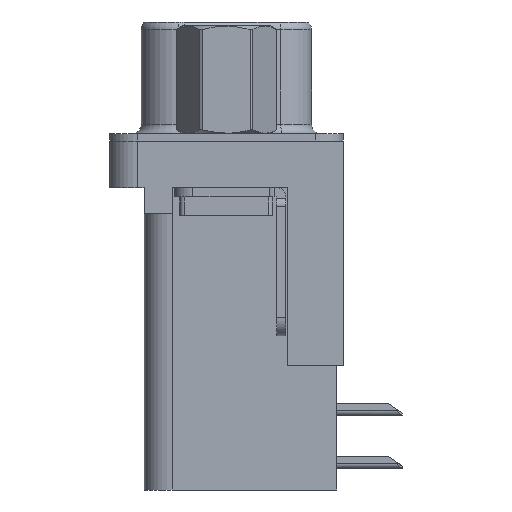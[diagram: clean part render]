
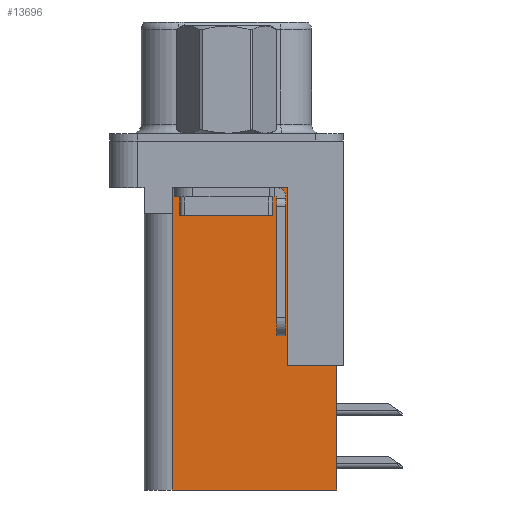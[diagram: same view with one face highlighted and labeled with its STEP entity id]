
A CAD part, left-side view. The second image highlights one B-rep face of the part: STEP entity #13696.
In plain terms, the highlighted planar face has unit normal (-1, 0, 0).
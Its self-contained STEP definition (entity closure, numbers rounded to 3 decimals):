
#97 = LINE ( 'NONE', #12691, #3397 ) ;
#1376 = VERTEX_POINT ( 'NONE', #2705 ) ;
#1845 = VERTEX_POINT ( 'NONE', #11958 ) ;
#1956 = VERTEX_POINT ( 'NONE', #14545 ) ;
#2577 = LINE ( 'NONE', #13006, #15642 ) ;
#2705 = CARTESIAN_POINT ( 'NONE',  ( 3.79, 2.895, -3.9 ) ) ;
#2809 = EDGE_CURVE ( 'NONE', #5071, #7004, #20610, .T. ) ;
#2997 = ORIENTED_EDGE ( 'NONE', *, *, #13222, .F. ) ;
#3215 = DIRECTION ( 'NONE',  ( 0., 1., 0. ) ) ;
#3397 = VECTOR ( 'NONE', #12629, 1000. ) ;
#3587 = DIRECTION ( 'NONE',  ( 0., 1., 0. ) ) ;
#3687 = VECTOR ( 'NONE', #3587, 1000. ) ;
#3914 = EDGE_LOOP ( 'NONE', ( #12178, #21031, #17771, #6407, #14233, #2997, #8395, #11514 ) ) ;
#4677 = CARTESIAN_POINT ( 'NONE',  ( 3.79, 2.895, -2.5 ) ) ;
#5071 = VERTEX_POINT ( 'NONE', #7408 ) ;
#5511 = CARTESIAN_POINT ( 'NONE',  ( 3.79, 2.895, -3.9 ) ) ;
#6101 = EDGE_CURVE ( 'NONE', #1376, #9246, #16309, .T. ) ;
#6351 = FACE_OUTER_BOUND ( 'NONE', #3914, .T. ) ;
#6407 = ORIENTED_EDGE ( 'NONE', *, *, #8198, .F. ) ;
#6561 = DIRECTION ( 'NONE',  ( 0., 1., 0. ) ) ;
#7004 = VERTEX_POINT ( 'NONE', #8080 ) ;
#7408 = CARTESIAN_POINT ( 'NONE',  ( 3.79, -5.925, -12.05 ) ) ;
#8080 = CARTESIAN_POINT ( 'NONE',  ( 3.79, -3.295, -12.05 ) ) ;
#8096 = DIRECTION ( 'NONE',  ( 1., 0., 0. ) ) ;
#8198 = EDGE_CURVE ( 'NONE', #1845, #9246, #13965, .T. ) ;
#8395 = ORIENTED_EDGE ( 'NONE', *, *, #2809, .T. ) ;
#8582 = VECTOR ( 'NONE', #15239, 1000. ) ;
#8687 = LINE ( 'NONE', #11045, #17398 ) ;
#8912 = EDGE_CURVE ( 'NONE', #16804, #1376, #14454, .T. ) ;
#8977 = CARTESIAN_POINT ( 'NONE',  ( 3.79, -3.295, -18.76 ) ) ;
#9246 = VERTEX_POINT ( 'NONE', #16480 ) ;
#9531 = DIRECTION ( 'NONE',  ( 0., 0., 1. ) ) ;
#9613 = VECTOR ( 'NONE', #9531, 1000. ) ;
#10152 = EDGE_CURVE ( 'NONE', #1956, #16804, #97, .T. ) ;
#10228 = LINE ( 'NONE', #8977, #14593 ) ;
#11045 = CARTESIAN_POINT ( 'NONE',  ( 3.79, -5.925, -2. ) ) ;
#11514 = ORIENTED_EDGE ( 'NONE', *, *, #15860, .T. ) ;
#11958 = CARTESIAN_POINT ( 'NONE',  ( 3.79, 2.925, -18.76 ) ) ;
#12178 = ORIENTED_EDGE ( 'NONE', *, *, #10152, .T. ) ;
#12629 = DIRECTION ( 'NONE',  ( 0., 1., 0. ) ) ;
#12691 = CARTESIAN_POINT ( 'NONE',  ( 3.79, -3.295, -2.5 ) ) ;
#12939 = PLANE ( 'NONE',  #15094 ) ;
#13006 = CARTESIAN_POINT ( 'NONE',  ( 3.79, -3.295, -18.76 ) ) ;
#13222 = EDGE_CURVE ( 'NONE', #5071, #17229, #8687, .T. ) ;
#13621 = CARTESIAN_POINT ( 'NONE',  ( 3.79, -6.295, -12.05 ) ) ;
#13696 = ADVANCED_FACE ( 'NONE', ( #6351 ), #12939, .F. ) ;
#13900 = DIRECTION ( 'NONE',  ( 0., 0., 1. ) ) ;
#13965 = LINE ( 'NONE', #14397, #9613 ) ;
#14233 = ORIENTED_EDGE ( 'NONE', *, *, #14265, .F. ) ;
#14265 = EDGE_CURVE ( 'NONE', #17229, #1845, #2577, .T. ) ;
#14397 = CARTESIAN_POINT ( 'NONE',  ( 3.79, 2.925, -18.76 ) ) ;
#14454 = LINE ( 'NONE', #5511, #8582 ) ;
#14545 = CARTESIAN_POINT ( 'NONE',  ( 3.79, -3.295, -2.5 ) ) ;
#14593 = VECTOR ( 'NONE', #13900, 1000. ) ;
#14959 = CARTESIAN_POINT ( 'NONE',  ( 3.79, -5.925, -18.76 ) ) ;
#15094 = AXIS2_PLACEMENT_3D ( 'NONE', #17922, #8096, #19574 ) ;
#15239 = DIRECTION ( 'NONE',  ( 0., 0., -1. ) ) ;
#15642 = VECTOR ( 'NONE', #3215, 1000. ) ;
#15860 = EDGE_CURVE ( 'NONE', #7004, #1956, #10228, .T. ) ;
#16309 = LINE ( 'NONE', #16378, #16820 ) ;
#16378 = CARTESIAN_POINT ( 'NONE',  ( 3.79, 0., -3.9 ) ) ;
#16480 = CARTESIAN_POINT ( 'NONE',  ( 3.79, 2.925, -3.9 ) ) ;
#16804 = VERTEX_POINT ( 'NONE', #4677 ) ;
#16820 = VECTOR ( 'NONE', #6561, 1000. ) ;
#17229 = VERTEX_POINT ( 'NONE', #14959 ) ;
#17398 = VECTOR ( 'NONE', #20874, 1000. ) ;
#17771 = ORIENTED_EDGE ( 'NONE', *, *, #6101, .T. ) ;
#17922 = CARTESIAN_POINT ( 'NONE',  ( 3.79, -3.295, -18.76 ) ) ;
#19574 = DIRECTION ( 'NONE',  ( 0., 1., 0. ) ) ;
#20610 = LINE ( 'NONE', #13621, #3687 ) ;
#20874 = DIRECTION ( 'NONE',  ( 0., 0., -1. ) ) ;
#21031 = ORIENTED_EDGE ( 'NONE', *, *, #8912, .T. ) ;
